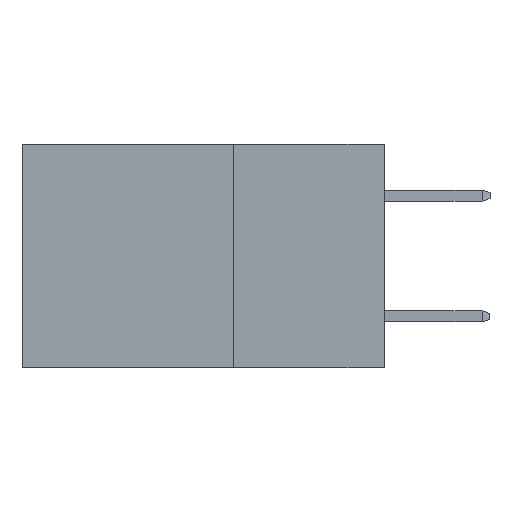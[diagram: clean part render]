
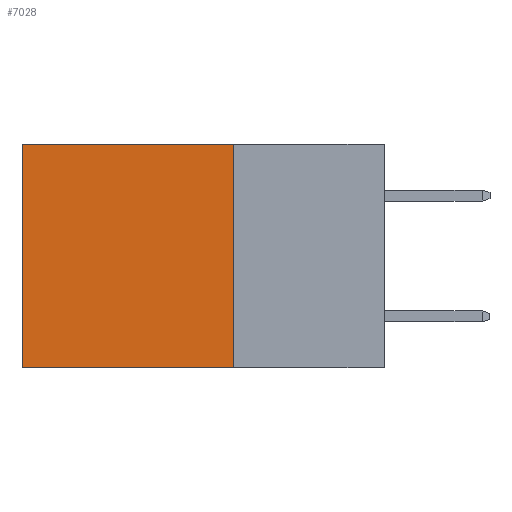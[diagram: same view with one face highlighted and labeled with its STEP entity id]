
A CAD part, left-side view. The second image highlights one B-rep face of the part: STEP entity #7028.
In plain terms, the highlighted planar face has unit normal (-1, 0, 0).
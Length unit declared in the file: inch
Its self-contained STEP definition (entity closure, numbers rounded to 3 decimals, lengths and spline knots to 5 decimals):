
#199 = DIRECTION ( 'NONE',  ( 1., 0., 0. ) ) ;
#874 = CARTESIAN_POINT ( 'NONE',  ( 0.298, 0.6, 0. ) ) ;
#1098 = VERTEX_POINT ( 'NONE', #8872 ) ;
#1128 = ORIENTED_EDGE ( 'NONE', *, *, #3091, .F. ) ;
#1315 = VECTOR ( 'NONE', #5542, 39.37008 ) ;
#2271 = DIRECTION ( 'NONE',  ( 0., 0., -1. ) ) ;
#2432 = VECTOR ( 'NONE', #3885, 39.37008 ) ;
#3091 = EDGE_CURVE ( 'NONE', #5588, #7877, #6497, .T. ) ;
#3390 = VERTEX_POINT ( 'NONE', #15726 ) ;
#3502 = CARTESIAN_POINT ( 'NONE',  ( 0.298, 0.25, -0.37 ) ) ;
#3885 = DIRECTION ( 'NONE',  ( 0., 1., 0. ) ) ;
#4010 = ORIENTED_EDGE ( 'NONE', *, *, #13738, .T. ) ;
#4028 = EDGE_CURVE ( 'NONE', #5588, #1098, #13112, .T. ) ;
#4322 = EDGE_CURVE ( 'NONE', #7877, #3390, #4948, .T. ) ;
#4340 = CARTESIAN_POINT ( 'NONE',  ( 0.298, 0.25, 0. ) ) ;
#4948 = LINE ( 'NONE', #3502, #1315 ) ;
#5542 = DIRECTION ( 'NONE',  ( 0., 1., 0. ) ) ;
#5588 = VERTEX_POINT ( 'NONE', #6239 ) ;
#6239 = CARTESIAN_POINT ( 'NONE',  ( 0.298, 0.25, 0. ) ) ;
#6383 = LINE ( 'NONE', #874, #13027 ) ;
#6497 = LINE ( 'NONE', #13654, #13141 ) ;
#7028 = ADVANCED_FACE ( 'NONE', ( #15353 ), #15627, .F. ) ;
#7161 = DIRECTION ( 'NONE',  ( 0., 0., -1. ) ) ;
#7877 = VERTEX_POINT ( 'NONE', #10323 ) ;
#8709 = EDGE_LOOP ( 'NONE', ( #4010, #11108, #1128, #10806 ) ) ;
#8872 = CARTESIAN_POINT ( 'NONE',  ( 0.298, 0.6, 0. ) ) ;
#10323 = CARTESIAN_POINT ( 'NONE',  ( 0.298, 0.25, -0.37 ) ) ;
#10806 = ORIENTED_EDGE ( 'NONE', *, *, #4028, .T. ) ;
#11108 = ORIENTED_EDGE ( 'NONE', *, *, #4322, .F. ) ;
#11358 = AXIS2_PLACEMENT_3D ( 'NONE', #14514, #199, #14701 ) ;
#13027 = VECTOR ( 'NONE', #2271, 39.37008 ) ;
#13112 = LINE ( 'NONE', #4340, #2432 ) ;
#13141 = VECTOR ( 'NONE', #7161, 39.37008 ) ;
#13654 = CARTESIAN_POINT ( 'NONE',  ( 0.298, 0.25, 0. ) ) ;
#13738 = EDGE_CURVE ( 'NONE', #1098, #3390, #6383, .T. ) ;
#14514 = CARTESIAN_POINT ( 'NONE',  ( 0.298, 0.25, 0. ) ) ;
#14701 = DIRECTION ( 'NONE',  ( 0., 0., -1. ) ) ;
#15353 = FACE_OUTER_BOUND ( 'NONE', #8709, .T. ) ;
#15627 = PLANE ( 'NONE',  #11358 ) ;
#15726 = CARTESIAN_POINT ( 'NONE',  ( 0.298, 0.6, -0.37 ) ) ;
